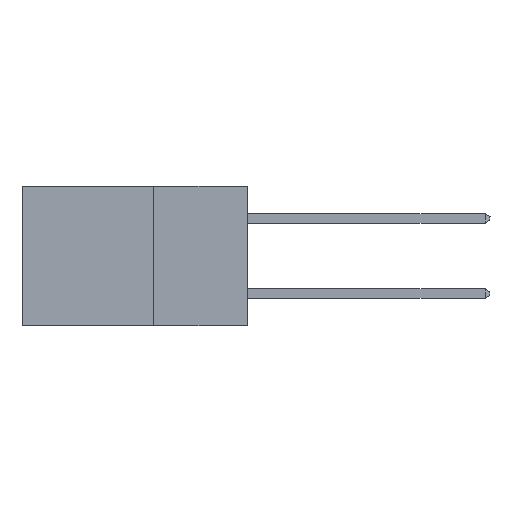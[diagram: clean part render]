
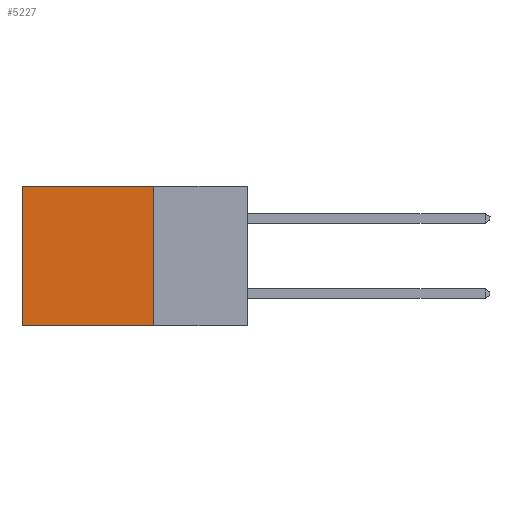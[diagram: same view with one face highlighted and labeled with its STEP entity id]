
A CAD part, left-side view. The second image highlights one B-rep face of the part: STEP entity #5227.
In plain terms, the highlighted planar face has unit normal (-1, 0, 0).
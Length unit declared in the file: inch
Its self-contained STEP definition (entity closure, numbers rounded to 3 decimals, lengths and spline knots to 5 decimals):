
#328 = LINE ( 'NONE', #16049, #13455 ) ;
#355 = VECTOR ( 'NONE', #1982, 39.37008 ) ;
#709 = VECTOR ( 'NONE', #7622, 39.37008 ) ;
#764 = LINE ( 'NONE', #10761, #355 ) ;
#852 = VERTEX_POINT ( 'NONE', #11938 ) ;
#1982 = DIRECTION ( 'NONE',  ( 0., 1., 0. ) ) ;
#2194 = EDGE_CURVE ( 'NONE', #852, #6529, #328, .T. ) ;
#2374 = AXIS2_PLACEMENT_3D ( 'NONE', #3520, #12392, #13655 ) ;
#2517 = CARTESIAN_POINT ( 'NONE',  ( 0.298, 0.25, 0. ) ) ;
#3248 = CARTESIAN_POINT ( 'NONE',  ( 0.298, 0.25, 0. ) ) ;
#3520 = CARTESIAN_POINT ( 'NONE',  ( 0.298, 0.25, 0. ) ) ;
#4229 = EDGE_LOOP ( 'NONE', ( #8766, #14669, #4667, #10014 ) ) ;
#4602 = VECTOR ( 'NONE', #13557, 39.37008 ) ;
#4667 = ORIENTED_EDGE ( 'NONE', *, *, #11917, .F. ) ;
#5227 = ADVANCED_FACE ( 'NONE', ( #14534 ), #5947, .F. ) ;
#5800 = CARTESIAN_POINT ( 'NONE',  ( 0.298, 0.25, 0. ) ) ;
#5947 = PLANE ( 'NONE',  #2374 ) ;
#6529 = VERTEX_POINT ( 'NONE', #12854 ) ;
#7622 = DIRECTION ( 'NONE',  ( 0., 0., -1. ) ) ;
#8228 = EDGE_CURVE ( 'NONE', #14470, #852, #16134, .T. ) ;
#8766 = ORIENTED_EDGE ( 'NONE', *, *, #2194, .T. ) ;
#9641 = LINE ( 'NONE', #5800, #709 ) ;
#10014 = ORIENTED_EDGE ( 'NONE', *, *, #8228, .T. ) ;
#10099 = CARTESIAN_POINT ( 'NONE',  ( 0.298, 0.25, -0.37 ) ) ;
#10761 = CARTESIAN_POINT ( 'NONE',  ( 0.298, 0.25, -0.37 ) ) ;
#11917 = EDGE_CURVE ( 'NONE', #14470, #12502, #9641, .T. ) ;
#11938 = CARTESIAN_POINT ( 'NONE',  ( 0.298, 0.6, 0. ) ) ;
#12091 = EDGE_CURVE ( 'NONE', #12502, #6529, #764, .T. ) ;
#12392 = DIRECTION ( 'NONE',  ( 1., 0., 0. ) ) ;
#12502 = VERTEX_POINT ( 'NONE', #10099 ) ;
#12854 = CARTESIAN_POINT ( 'NONE',  ( 0.298, 0.6, -0.37 ) ) ;
#13455 = VECTOR ( 'NONE', #14821, 39.37008 ) ;
#13557 = DIRECTION ( 'NONE',  ( 0., 1., 0. ) ) ;
#13655 = DIRECTION ( 'NONE',  ( 0., 0., -1. ) ) ;
#14470 = VERTEX_POINT ( 'NONE', #2517 ) ;
#14534 = FACE_OUTER_BOUND ( 'NONE', #4229, .T. ) ;
#14669 = ORIENTED_EDGE ( 'NONE', *, *, #12091, .F. ) ;
#14821 = DIRECTION ( 'NONE',  ( 0., 0., -1. ) ) ;
#16049 = CARTESIAN_POINT ( 'NONE',  ( 0.298, 0.6, 0. ) ) ;
#16134 = LINE ( 'NONE', #3248, #4602 ) ;
